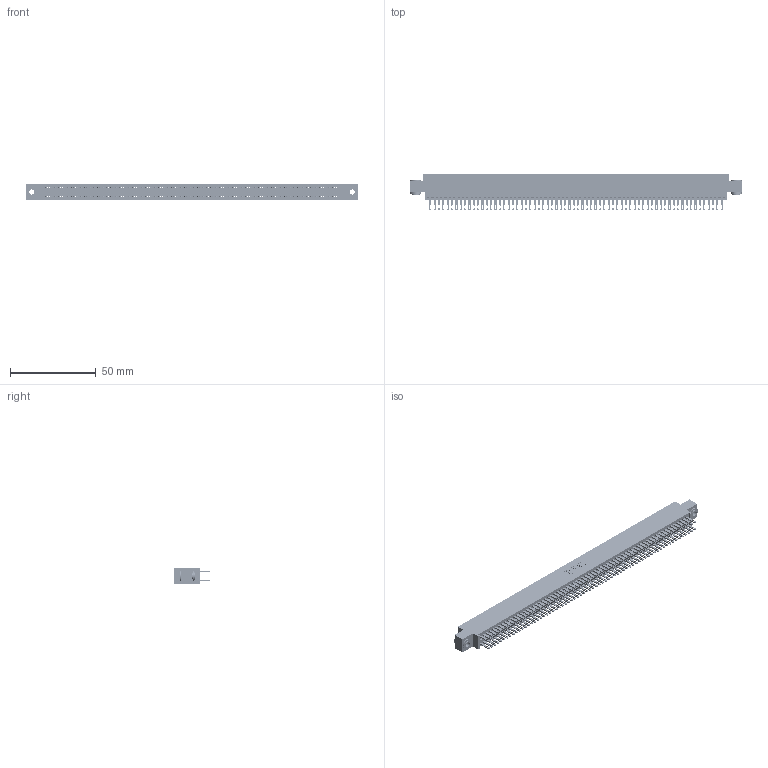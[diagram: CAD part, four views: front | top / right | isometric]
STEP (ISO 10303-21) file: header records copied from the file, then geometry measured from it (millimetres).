
FILE_DESCRIPTION (( 'STEP AP203' ), '1' );
FILE_NAME ('895-136-500-803.STEP', '2020-10-13T18:36:03', ( '' ), ( '' ), 'SwSTEP 2.0', 'SolidWorks 2020', '' );
FILE_SCHEMA (( 'CONFIG_CONTROL_DESIGN' ));
Length unit declared in the file: inch
Products named in the file (4): 895-136-500-803; 345-292-001_345-293-100; 845 Part_0.170 Offset - 0.156 Dia-TH; 345-250-002_345-250-002-102
Assembly tree (139 placements, depth 2):
  895-136-500-803
    845 Part_0.170 Offset - 0.156 Dia-TH
    345-292-001_345-293-100  x136
    345-250-002_345-250-002-102  x2
Bounding box: 193.93 x 21.51 x 9.4 mm (x, y, z)
Volume: 19401.4 mm3; surface area: 30917.6 mm2
Topology: 139 solids, 139 shells, 6424 faces, 19605 edges, 13066 vertices
Faces by surface type: plane 3766, cylinder 2650, cone 8
Entity records: 50566 total; most frequent: CARTESIAN_POINT 8427, ORIENTED_EDGE 8354, DIRECTION 7431, EDGE_CURVE 4177, VECTOR 3745, LINE 3745, VERTEX_POINT 2782, AXIS2_PLACEMENT_3D 1843
